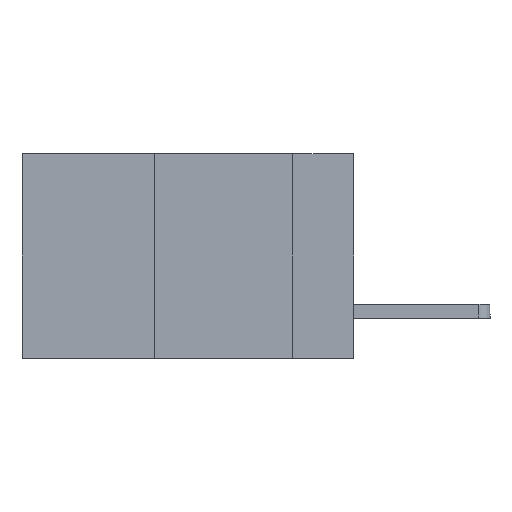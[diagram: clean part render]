
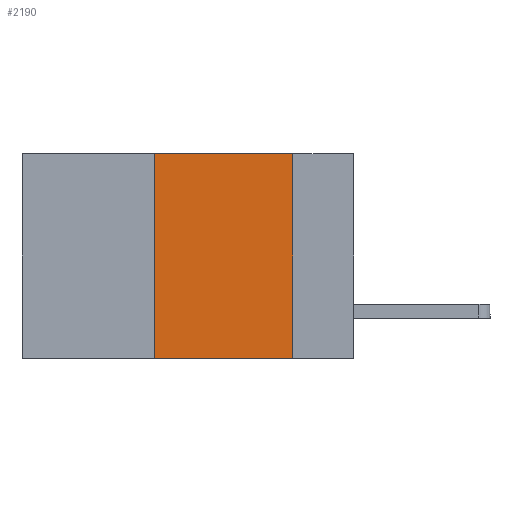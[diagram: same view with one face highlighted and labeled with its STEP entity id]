
A CAD part, left-side view. The second image highlights one B-rep face of the part: STEP entity #2190.
In plain terms, the highlighted planar face has unit normal (-1, 0, 0).
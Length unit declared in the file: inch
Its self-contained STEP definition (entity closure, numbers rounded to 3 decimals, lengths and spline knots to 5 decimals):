
#187 = DIRECTION ( 'NONE',  ( 0., 0., 1. ) ) ;
#274 = EDGE_LOOP ( 'NONE', ( #8674, #3405, #3511, #5765 ) ) ;
#324 = DIRECTION ( 'NONE',  ( 1., 0., 0. ) ) ;
#458 = EDGE_CURVE ( 'NONE', #4609, #9233, #3560, .T. ) ;
#1202 = EDGE_CURVE ( 'NONE', #9233, #4404, #8643, .T. ) ;
#1248 = DIRECTION ( 'NONE',  ( 0., -1., 0. ) ) ;
#1440 = VERTEX_POINT ( 'NONE', #7774 ) ;
#1943 = CARTESIAN_POINT ( 'NONE',  ( 0., 0.6, -0.37 ) ) ;
#2190 = ADVANCED_FACE ( 'NONE', ( #6801 ), #3403, .F. ) ;
#2240 = VECTOR ( 'NONE', #4850, 39.37008 ) ;
#3403 = PLANE ( 'NONE',  #8188 ) ;
#3405 = ORIENTED_EDGE ( 'NONE', *, *, #1202, .F. ) ;
#3511 = ORIENTED_EDGE ( 'NONE', *, *, #458, .F. ) ;
#3560 = LINE ( 'NONE', #5370, #9734 ) ;
#4166 = CARTESIAN_POINT ( 'NONE',  ( 0., 0.6, 0. ) ) ;
#4404 = VERTEX_POINT ( 'NONE', #9216 ) ;
#4609 = VERTEX_POINT ( 'NONE', #5635 ) ;
#4620 = EDGE_CURVE ( 'NONE', #4404, #1440, #8182, .T. ) ;
#4850 = DIRECTION ( 'NONE',  ( 0., 0., -1. ) ) ;
#5370 = CARTESIAN_POINT ( 'NONE',  ( 0., 0.36, 0. ) ) ;
#5553 = LINE ( 'NONE', #1943, #5806 ) ;
#5635 = CARTESIAN_POINT ( 'NONE',  ( 0., 0.36, -0.37 ) ) ;
#5759 = DIRECTION ( 'NONE',  ( 0., 0., -1. ) ) ;
#5765 = ORIENTED_EDGE ( 'NONE', *, *, #9156, .T. ) ;
#5806 = VECTOR ( 'NONE', #7391, 39.37008 ) ;
#6801 = FACE_OUTER_BOUND ( 'NONE', #274, .T. ) ;
#6844 = VECTOR ( 'NONE', #1248, 39.37008 ) ;
#7391 = DIRECTION ( 'NONE',  ( 0., -1., 0. ) ) ;
#7774 = CARTESIAN_POINT ( 'NONE',  ( 0., 0.11, -0.37 ) ) ;
#8182 = LINE ( 'NONE', #9477, #2240 ) ;
#8188 = AXIS2_PLACEMENT_3D ( 'NONE', #4166, #324, #5759 ) ;
#8233 = CARTESIAN_POINT ( 'NONE',  ( 0., 0.6, 0. ) ) ;
#8643 = LINE ( 'NONE', #8233, #6844 ) ;
#8674 = ORIENTED_EDGE ( 'NONE', *, *, #4620, .F. ) ;
#9156 = EDGE_CURVE ( 'NONE', #4609, #1440, #5553, .T. ) ;
#9216 = CARTESIAN_POINT ( 'NONE',  ( 0., 0.11, 0. ) ) ;
#9233 = VERTEX_POINT ( 'NONE', #9768 ) ;
#9477 = CARTESIAN_POINT ( 'NONE',  ( 0., 0.11, 0. ) ) ;
#9734 = VECTOR ( 'NONE', #187, 39.37008 ) ;
#9768 = CARTESIAN_POINT ( 'NONE',  ( 0., 0.36, 0. ) ) ;
